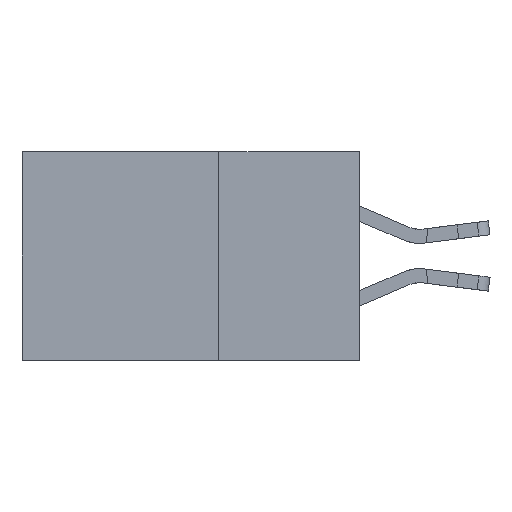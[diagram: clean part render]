
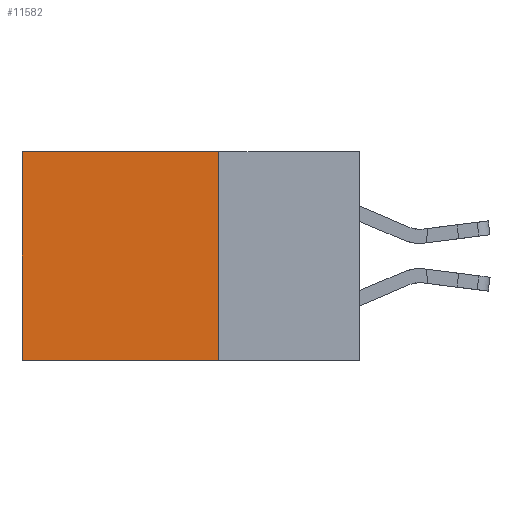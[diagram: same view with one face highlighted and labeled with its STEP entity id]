
A CAD part, left-side view. The second image highlights one B-rep face of the part: STEP entity #11582.
In plain terms, the highlighted planar face has unit normal (-1, 0, 0).
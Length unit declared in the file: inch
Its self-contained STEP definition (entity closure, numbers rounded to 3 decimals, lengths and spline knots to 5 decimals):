
#172 = LINE ( 'NONE', #9334, #952 ) ;
#388 = CARTESIAN_POINT ( 'NONE',  ( 0.2875, 0.6, -0.37 ) ) ;
#637 = CARTESIAN_POINT ( 'NONE',  ( 0.2875, 0.25, 0. ) ) ;
#856 = LINE ( 'NONE', #1968, #10670 ) ;
#952 = VECTOR ( 'NONE', #4495, 39.37008 ) ;
#990 = EDGE_CURVE ( 'NONE', #17561, #19270, #172, .T. ) ;
#1747 = CARTESIAN_POINT ( 'NONE',  ( 0.2875, 0.25, 0. ) ) ;
#1968 = CARTESIAN_POINT ( 'NONE',  ( 0.2875, 0.25, 0. ) ) ;
#2030 = ORIENTED_EDGE ( 'NONE', *, *, #990, .F. ) ;
#2535 = FACE_OUTER_BOUND ( 'NONE', #10628, .T. ) ;
#2776 = AXIS2_PLACEMENT_3D ( 'NONE', #11233, #12774, #14700 ) ;
#3523 = DIRECTION ( 'NONE',  ( 0., 0., -1. ) ) ;
#4495 = DIRECTION ( 'NONE',  ( 0., 1., 0. ) ) ;
#7295 = DIRECTION ( 'NONE',  ( 0., 0., -1. ) ) ;
#8132 = PLANE ( 'NONE',  #2776 ) ;
#8990 = VECTOR ( 'NONE', #11125, 39.37008 ) ;
#9334 = CARTESIAN_POINT ( 'NONE',  ( 0.2875, 0.25, -0.37 ) ) ;
#9436 = VECTOR ( 'NONE', #7295, 39.37008 ) ;
#10628 = EDGE_LOOP ( 'NONE', ( #12375, #2030, #11194, #12747 ) ) ;
#10670 = VECTOR ( 'NONE', #3523, 39.37008 ) ;
#11125 = DIRECTION ( 'NONE',  ( 0., 1., 0. ) ) ;
#11194 = ORIENTED_EDGE ( 'NONE', *, *, #16004, .F. ) ;
#11233 = CARTESIAN_POINT ( 'NONE',  ( 0.2875, 0.25, 0. ) ) ;
#11582 = ADVANCED_FACE ( 'NONE', ( #2535 ), #8132, .F. ) ;
#11950 = EDGE_CURVE ( 'NONE', #13271, #19979, #20065, .T. ) ;
#12375 = ORIENTED_EDGE ( 'NONE', *, *, #15326, .T. ) ;
#12747 = ORIENTED_EDGE ( 'NONE', *, *, #11950, .T. ) ;
#12774 = DIRECTION ( 'NONE',  ( 1., 0., 0. ) ) ;
#13271 = VERTEX_POINT ( 'NONE', #637 ) ;
#13539 = CARTESIAN_POINT ( 'NONE',  ( 0.2875, 0.6, 0. ) ) ;
#14700 = DIRECTION ( 'NONE',  ( 0., 0., -1. ) ) ;
#15326 = EDGE_CURVE ( 'NONE', #19979, #19270, #20046, .T. ) ;
#16004 = EDGE_CURVE ( 'NONE', #13271, #17561, #856, .T. ) ;
#16263 = CARTESIAN_POINT ( 'NONE',  ( 0.2875, 0.6, 0. ) ) ;
#16623 = CARTESIAN_POINT ( 'NONE',  ( 0.2875, 0.25, -0.37 ) ) ;
#17561 = VERTEX_POINT ( 'NONE', #16623 ) ;
#19270 = VERTEX_POINT ( 'NONE', #388 ) ;
#19979 = VERTEX_POINT ( 'NONE', #16263 ) ;
#20046 = LINE ( 'NONE', #13539, #9436 ) ;
#20065 = LINE ( 'NONE', #1747, #8990 ) ;
